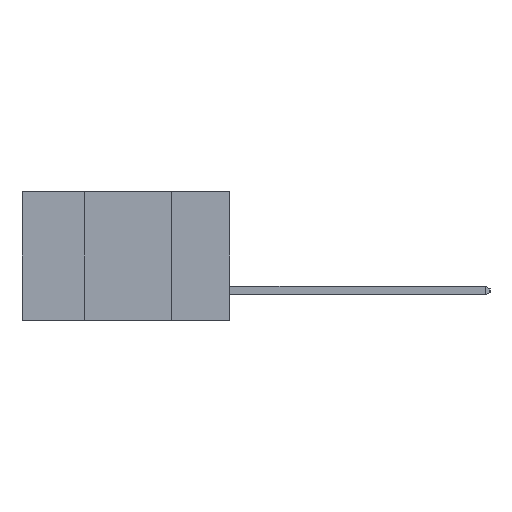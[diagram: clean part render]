
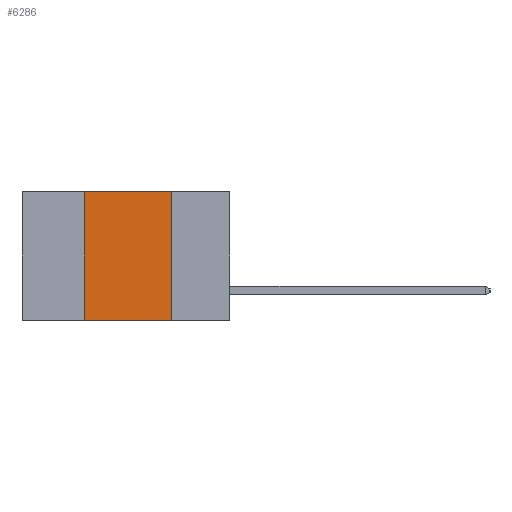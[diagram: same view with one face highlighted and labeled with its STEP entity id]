
A CAD part, left-side view. The second image highlights one B-rep face of the part: STEP entity #6286.
In plain terms, the highlighted planar face has unit normal (-1, 0, 0).
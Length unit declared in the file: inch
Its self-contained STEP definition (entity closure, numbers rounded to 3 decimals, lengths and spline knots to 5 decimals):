
#463 = CARTESIAN_POINT ( 'NONE',  ( 0., 0.42, -0.37 ) ) ;
#632 = ORIENTED_EDGE ( 'NONE', *, *, #11271, .T. ) ;
#823 = PLANE ( 'NONE',  #13438 ) ;
#879 = CARTESIAN_POINT ( 'NONE',  ( 0., 0.6, 0. ) ) ;
#1330 = ORIENTED_EDGE ( 'NONE', *, *, #9644, .F. ) ;
#1955 = DIRECTION ( 'NONE',  ( 0., 0., -1. ) ) ;
#1970 = DIRECTION ( 'NONE',  ( 1., 0., 0. ) ) ;
#2195 = CARTESIAN_POINT ( 'NONE',  ( 0., 0.17, 0. ) ) ;
#2954 = ORIENTED_EDGE ( 'NONE', *, *, #15239, .F. ) ;
#2965 = VERTEX_POINT ( 'NONE', #7972 ) ;
#3518 = ORIENTED_EDGE ( 'NONE', *, *, #12082, .F. ) ;
#3739 = CARTESIAN_POINT ( 'NONE',  ( 0., 0.42, -0.37 ) ) ;
#6016 = LINE ( 'NONE', #14419, #8928 ) ;
#6286 = ADVANCED_FACE ( 'NONE', ( #6295 ), #823, .F. ) ;
#6295 = FACE_OUTER_BOUND ( 'NONE', #14467, .T. ) ;
#6565 = DIRECTION ( 'NONE',  ( 0., -1., 0. ) ) ;
#6761 = LINE ( 'NONE', #12509, #9638 ) ;
#7186 = VECTOR ( 'NONE', #12363, 39.37008 ) ;
#7972 = CARTESIAN_POINT ( 'NONE',  ( 0., 0.17, -0.37 ) ) ;
#8041 = CARTESIAN_POINT ( 'NONE',  ( 0., 0.42, 0. ) ) ;
#8928 = VECTOR ( 'NONE', #15627, 39.37008 ) ;
#9638 = VECTOR ( 'NONE', #13645, 39.37008 ) ;
#9644 = EDGE_CURVE ( 'NONE', #12305, #12294, #13630, .T. ) ;
#10644 = VERTEX_POINT ( 'NONE', #2195 ) ;
#11271 = EDGE_CURVE ( 'NONE', #12305, #2965, #6016, .T. ) ;
#12018 = VECTOR ( 'NONE', #6565, 39.37008 ) ;
#12082 = EDGE_CURVE ( 'NONE', #10644, #2965, #6761, .T. ) ;
#12294 = VERTEX_POINT ( 'NONE', #8041 ) ;
#12305 = VERTEX_POINT ( 'NONE', #463 ) ;
#12363 = DIRECTION ( 'NONE',  ( 0., 0., 1. ) ) ;
#12509 = CARTESIAN_POINT ( 'NONE',  ( 0., 0.17, -0.37 ) ) ;
#12655 = CARTESIAN_POINT ( 'NONE',  ( 0., 0.6, 0. ) ) ;
#13438 = AXIS2_PLACEMENT_3D ( 'NONE', #879, #1970, #1955 ) ;
#13630 = LINE ( 'NONE', #3739, #7186 ) ;
#13645 = DIRECTION ( 'NONE',  ( 0., 0., -1. ) ) ;
#14419 = CARTESIAN_POINT ( 'NONE',  ( 0., 0.6, -0.37 ) ) ;
#14467 = EDGE_LOOP ( 'NONE', ( #3518, #2954, #1330, #632 ) ) ;
#15138 = LINE ( 'NONE', #12655, #12018 ) ;
#15239 = EDGE_CURVE ( 'NONE', #12294, #10644, #15138, .T. ) ;
#15627 = DIRECTION ( 'NONE',  ( 0., -1., 0. ) ) ;
